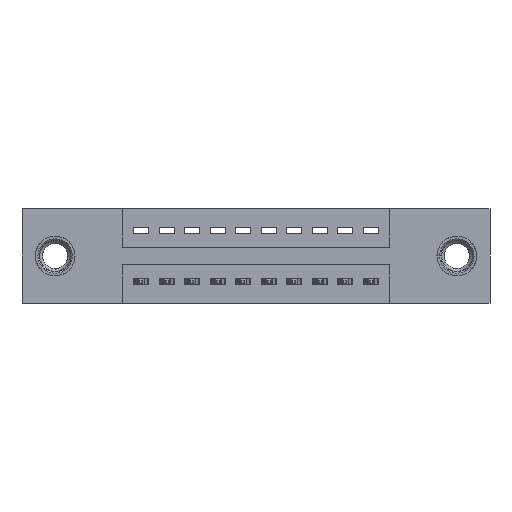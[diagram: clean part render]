
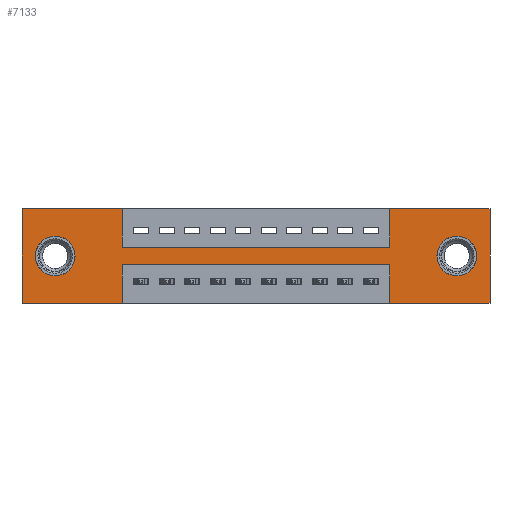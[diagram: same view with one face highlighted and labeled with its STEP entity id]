
A CAD part, front view. The second image highlights one B-rep face of the part: STEP entity #7133.
In plain terms, the highlighted planar face has unit normal (0, -1, 0).
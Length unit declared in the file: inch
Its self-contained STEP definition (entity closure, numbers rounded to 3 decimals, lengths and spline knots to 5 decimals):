
#21 = CARTESIAN_POINT ( 'NONE',  ( 0.3925, 0., -0.15 ) ) ;
#95 = VERTEX_POINT ( 'NONE', #11961 ) ;
#215 = ORIENTED_EDGE ( 'NONE', *, *, #4278, .F. ) ;
#335 = CARTESIAN_POINT ( 'NONE',  ( 0.3925, 0., -0.22 ) ) ;
#383 = DIRECTION ( 'NONE',  ( 0., 0., 1. ) ) ;
#398 = CIRCLE ( 'NONE', #7845, 0.078 ) ;
#403 = EDGE_CURVE ( 'NONE', #9005, #4078, #10031, .T. ) ;
#438 = LINE ( 'NONE', #12930, #3141 ) ;
#541 = CARTESIAN_POINT ( 'NONE',  ( 1.4425, 0., -0.37 ) ) ;
#630 = CARTESIAN_POINT ( 'NONE',  ( 0., 0., -0.37 ) ) ;
#776 = VECTOR ( 'NONE', #5914, 39.37008 ) ;
#870 = CARTESIAN_POINT ( 'NONE',  ( 1.705, 0., -0.185 ) ) ;
#878 = DIRECTION ( 'NONE',  ( 0., 1., 0. ) ) ;
#950 = LINE ( 'NONE', #5933, #11352 ) ;
#1175 = CARTESIAN_POINT ( 'NONE',  ( 0.3925, 0., -0.37 ) ) ;
#1250 = LINE ( 'NONE', #8367, #6284 ) ;
#1269 = ORIENTED_EDGE ( 'NONE', *, *, #10800, .T. ) ;
#1288 = CARTESIAN_POINT ( 'NONE',  ( 1.4425, 0., -0.15 ) ) ;
#1374 = EDGE_CURVE ( 'NONE', #11547, #12715, #11885, .T. ) ;
#1446 = EDGE_CURVE ( 'NONE', #5013, #95, #398, .T. ) ;
#1611 = VERTEX_POINT ( 'NONE', #335 ) ;
#1673 = VERTEX_POINT ( 'NONE', #4487 ) ;
#1708 = DIRECTION ( 'NONE',  ( 0., 0., -1. ) ) ;
#1709 = LINE ( 'NONE', #9921, #776 ) ;
#1759 = ORIENTED_EDGE ( 'NONE', *, *, #5431, .F. ) ;
#1772 = DIRECTION ( 'NONE',  ( 1., 0., 0. ) ) ;
#1872 = DIRECTION ( 'NONE',  ( 0., 0., -1. ) ) ;
#1876 = DIRECTION ( 'NONE',  ( -1., 0., 0. ) ) ;
#1949 = DIRECTION ( 'NONE',  ( 0., 0., -1. ) ) ;
#2421 = DIRECTION ( 'NONE',  ( -1., 0., 0. ) ) ;
#2595 = ORIENTED_EDGE ( 'NONE', *, *, #403, .F. ) ;
#2817 = VECTOR ( 'NONE', #6231, 39.37008 ) ;
#2860 = LINE ( 'NONE', #9842, #12906 ) ;
#2946 = ORIENTED_EDGE ( 'NONE', *, *, #3777, .F. ) ;
#3039 = CARTESIAN_POINT ( 'NONE',  ( 1.705, 0., -0.185 ) ) ;
#3040 = EDGE_LOOP ( 'NONE', ( #10199, #1269 ) ) ;
#3114 = DIRECTION ( 'NONE',  ( 0., 1., 0. ) ) ;
#3141 = VECTOR ( 'NONE', #9060, 39.37008 ) ;
#3304 = ORIENTED_EDGE ( 'NONE', *, *, #1374, .F. ) ;
#3445 = CARTESIAN_POINT ( 'NONE',  ( 1.4425, 0., 0. ) ) ;
#3446 = ORIENTED_EDGE ( 'NONE', *, *, #10603, .F. ) ;
#3494 = ORIENTED_EDGE ( 'NONE', *, *, #9646, .F. ) ;
#3777 = EDGE_CURVE ( 'NONE', #12715, #9005, #950, .T. ) ;
#4067 = LINE ( 'NONE', #21, #11750 ) ;
#4078 = VERTEX_POINT ( 'NONE', #541 ) ;
#4278 = EDGE_CURVE ( 'NONE', #8777, #8511, #1250, .T. ) ;
#4438 = CIRCLE ( 'NONE', #8524, 0.078 ) ;
#4487 = CARTESIAN_POINT ( 'NONE',  ( 1.4425, 0., -0.22 ) ) ;
#4542 = EDGE_CURVE ( 'NONE', #11364, #11547, #12720, .T. ) ;
#4559 = DIRECTION ( 'NONE',  ( 0., 0., -1. ) ) ;
#4707 = CARTESIAN_POINT ( 'NONE',  ( 1.835, 0., 0. ) ) ;
#4868 = EDGE_CURVE ( 'NONE', #4078, #1673, #438, .T. ) ;
#4901 = CARTESIAN_POINT ( 'NONE',  ( 0.13, 0., -0.185 ) ) ;
#5008 = CARTESIAN_POINT ( 'NONE',  ( 1.705, 0., -0.107 ) ) ;
#5013 = VERTEX_POINT ( 'NONE', #5502 ) ;
#5134 = FACE_BOUND ( 'NONE', #3040, .T. ) ;
#5223 = CARTESIAN_POINT ( 'NONE',  ( 1.835, 0., -0.37 ) ) ;
#5431 = EDGE_CURVE ( 'NONE', #8511, #11364, #4067, .T. ) ;
#5437 = FACE_BOUND ( 'NONE', #11470, .T. ) ;
#5502 = CARTESIAN_POINT ( 'NONE',  ( 0.13, 0., -0.107 ) ) ;
#5539 = VERTEX_POINT ( 'NONE', #10294 ) ;
#5888 = CARTESIAN_POINT ( 'NONE',  ( 0.3925, 0., -0.15 ) ) ;
#5914 = DIRECTION ( 'NONE',  ( 0., 0., 1. ) ) ;
#5933 = CARTESIAN_POINT ( 'NONE',  ( 1.835, 0., 0. ) ) ;
#6231 = DIRECTION ( 'NONE',  ( 1., 0., 0. ) ) ;
#6284 = VECTOR ( 'NONE', #4559, 39.37008 ) ;
#6412 = CIRCLE ( 'NONE', #7933, 0.078 ) ;
#6466 = AXIS2_PLACEMENT_3D ( 'NONE', #870, #7903, #1872 ) ;
#6832 = CARTESIAN_POINT ( 'NONE',  ( 0.3925, 0., 0. ) ) ;
#6840 = VERTEX_POINT ( 'NONE', #5008 ) ;
#6913 = ORIENTED_EDGE ( 'NONE', *, *, #12901, .T. ) ;
#6978 = VECTOR ( 'NONE', #1876, 39.37008 ) ;
#7098 = DIRECTION ( 'NONE',  ( 1., 0., 0. ) ) ;
#7133 = ADVANCED_FACE ( 'NONE', ( #5437, #5134, #7150 ), #8630, .T. ) ;
#7150 = FACE_OUTER_BOUND ( 'NONE', #9238, .T. ) ;
#7163 = CARTESIAN_POINT ( 'NONE',  ( 0.13, 0., -0.185 ) ) ;
#7183 = LINE ( 'NONE', #8082, #2817 ) ;
#7236 = VERTEX_POINT ( 'NONE', #630 ) ;
#7310 = LINE ( 'NONE', #10570, #6978 ) ;
#7455 = VERTEX_POINT ( 'NONE', #1175 ) ;
#7845 = AXIS2_PLACEMENT_3D ( 'NONE', #7163, #3114, #10092 ) ;
#7903 = DIRECTION ( 'NONE',  ( 0., 1., 0. ) ) ;
#7933 = AXIS2_PLACEMENT_3D ( 'NONE', #3039, #8903, #10053 ) ;
#8082 = CARTESIAN_POINT ( 'NONE',  ( 0., 0., 0. ) ) ;
#8140 = ORIENTED_EDGE ( 'NONE', *, *, #12442, .F. ) ;
#8367 = CARTESIAN_POINT ( 'NONE',  ( 0.3925, 0., 0. ) ) ;
#8511 = VERTEX_POINT ( 'NONE', #5888 ) ;
#8524 = AXIS2_PLACEMENT_3D ( 'NONE', #4901, #878, #12977 ) ;
#8551 = EDGE_CURVE ( 'NONE', #5539, #6840, #10740, .T. ) ;
#8630 = PLANE ( 'NONE',  #10179 ) ;
#8777 = VERTEX_POINT ( 'NONE', #6832 ) ;
#8802 = DIRECTION ( 'NONE',  ( 0., -1., 0. ) ) ;
#8843 = ORIENTED_EDGE ( 'NONE', *, *, #9816, .F. ) ;
#8884 = CARTESIAN_POINT ( 'NONE',  ( 0., 0., -0.37 ) ) ;
#8903 = DIRECTION ( 'NONE',  ( 0., 1., 0. ) ) ;
#9005 = VERTEX_POINT ( 'NONE', #5223 ) ;
#9060 = DIRECTION ( 'NONE',  ( 0., 0., 1. ) ) ;
#9201 = ORIENTED_EDGE ( 'NONE', *, *, #11743, .F. ) ;
#9220 = VECTOR ( 'NONE', #1772, 39.37008 ) ;
#9238 = EDGE_LOOP ( 'NONE', ( #9201, #3494, #12766, #2595, #2946, #3304, #10252, #1759, #215, #8140, #8843, #3446 ) ) ;
#9646 = EDGE_CURVE ( 'NONE', #1673, #1611, #2860, .T. ) ;
#9816 = EDGE_CURVE ( 'NONE', #7236, #10150, #1709, .T. ) ;
#9842 = CARTESIAN_POINT ( 'NONE',  ( 0.3925, 0., -0.22 ) ) ;
#9921 = CARTESIAN_POINT ( 'NONE',  ( 0., 0., 0. ) ) ;
#10031 = LINE ( 'NONE', #8884, #11450 ) ;
#10053 = DIRECTION ( 'NONE',  ( 0., 0., -1. ) ) ;
#10092 = DIRECTION ( 'NONE',  ( 0., 0., 1. ) ) ;
#10150 = VERTEX_POINT ( 'NONE', #12561 ) ;
#10179 = AXIS2_PLACEMENT_3D ( 'NONE', #12850, #8802, #1708 ) ;
#10199 = ORIENTED_EDGE ( 'NONE', *, *, #1446, .T. ) ;
#10252 = ORIENTED_EDGE ( 'NONE', *, *, #4542, .F. ) ;
#10294 = CARTESIAN_POINT ( 'NONE',  ( 1.705, 0., -0.263 ) ) ;
#10570 = CARTESIAN_POINT ( 'NONE',  ( 0., 0., -0.37 ) ) ;
#10603 = EDGE_CURVE ( 'NONE', #7455, #7236, #7310, .T. ) ;
#10675 = VECTOR ( 'NONE', #383, 39.37008 ) ;
#10710 = CARTESIAN_POINT ( 'NONE',  ( 1.4425, 0., 0. ) ) ;
#10740 = CIRCLE ( 'NONE', #6466, 0.078 ) ;
#10800 = EDGE_CURVE ( 'NONE', #95, #5013, #4438, .T. ) ;
#10829 = DIRECTION ( 'NONE',  ( -1., 0., 0. ) ) ;
#11163 = LINE ( 'NONE', #12822, #13050 ) ;
#11352 = VECTOR ( 'NONE', #12973, 39.37008 ) ;
#11364 = VERTEX_POINT ( 'NONE', #1288 ) ;
#11450 = VECTOR ( 'NONE', #10829, 39.37008 ) ;
#11470 = EDGE_LOOP ( 'NONE', ( #6913, #12034 ) ) ;
#11547 = VERTEX_POINT ( 'NONE', #10710 ) ;
#11743 = EDGE_CURVE ( 'NONE', #1611, #7455, #11163, .T. ) ;
#11750 = VECTOR ( 'NONE', #7098, 39.37008 ) ;
#11811 = CARTESIAN_POINT ( 'NONE',  ( 0., 0., 0. ) ) ;
#11885 = LINE ( 'NONE', #11811, #9220 ) ;
#11961 = CARTESIAN_POINT ( 'NONE',  ( 0.13, 0., -0.263 ) ) ;
#12034 = ORIENTED_EDGE ( 'NONE', *, *, #8551, .T. ) ;
#12442 = EDGE_CURVE ( 'NONE', #10150, #8777, #7183, .T. ) ;
#12561 = CARTESIAN_POINT ( 'NONE',  ( 0., 0., 0. ) ) ;
#12715 = VERTEX_POINT ( 'NONE', #4707 ) ;
#12720 = LINE ( 'NONE', #3445, #10675 ) ;
#12766 = ORIENTED_EDGE ( 'NONE', *, *, #4868, .F. ) ;
#12822 = CARTESIAN_POINT ( 'NONE',  ( 0.3925, 0., -0.37 ) ) ;
#12850 = CARTESIAN_POINT ( 'NONE',  ( 0., 0., -0.37 ) ) ;
#12901 = EDGE_CURVE ( 'NONE', #6840, #5539, #6412, .T. ) ;
#12906 = VECTOR ( 'NONE', #2421, 39.37008 ) ;
#12930 = CARTESIAN_POINT ( 'NONE',  ( 1.4425, 0., -0.37 ) ) ;
#12973 = DIRECTION ( 'NONE',  ( 0., 0., -1. ) ) ;
#12977 = DIRECTION ( 'NONE',  ( 0., 0., 1. ) ) ;
#13050 = VECTOR ( 'NONE', #1949, 39.37008 ) ;
